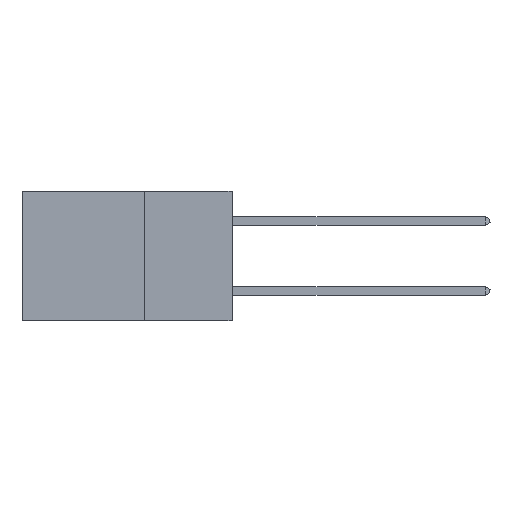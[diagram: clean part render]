
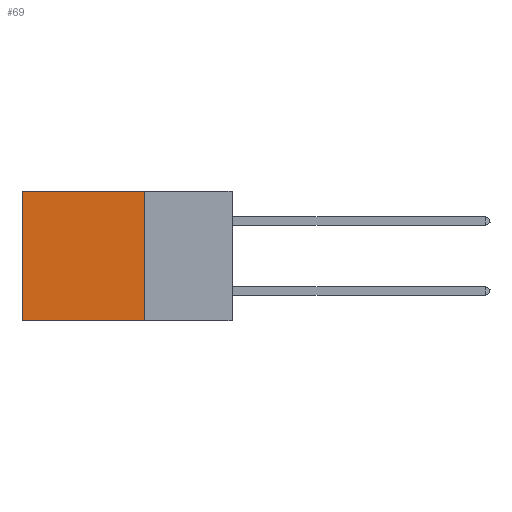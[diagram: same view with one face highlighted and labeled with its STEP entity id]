
A CAD part, left-side view. The second image highlights one B-rep face of the part: STEP entity #69.
In plain terms, the highlighted planar face has unit normal (-1, 0, 0).
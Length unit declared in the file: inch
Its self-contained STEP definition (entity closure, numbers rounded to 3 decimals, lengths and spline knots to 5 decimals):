
#69 = ADVANCED_FACE ( 'NONE', ( #638 ), #16818, .F. ) ;
#638 = FACE_OUTER_BOUND ( 'NONE', #28349, .T. ) ;
#1657 = VECTOR ( 'NONE', #23909, 39.37008 ) ;
#3343 = CARTESIAN_POINT ( 'NONE',  ( 0.2875, 0.25, -0.37 ) ) ;
#3465 = ORIENTED_EDGE ( 'NONE', *, *, #26536, .F. ) ;
#4228 = LINE ( 'NONE', #7484, #1657 ) ;
#5165 = EDGE_CURVE ( 'NONE', #7110, #7031, #12620, .T. ) ;
#7031 = VERTEX_POINT ( 'NONE', #13785 ) ;
#7110 = VERTEX_POINT ( 'NONE', #11536 ) ;
#7484 = CARTESIAN_POINT ( 'NONE',  ( 0.2875, 0.25, 0. ) ) ;
#7607 = ORIENTED_EDGE ( 'NONE', *, *, #5165, .T. ) ;
#9063 = ORIENTED_EDGE ( 'NONE', *, *, #27672, .F. ) ;
#9818 = AXIS2_PLACEMENT_3D ( 'NONE', #23804, #14626, #26576 ) ;
#10009 = DIRECTION ( 'NONE',  ( 0., 0., -1. ) ) ;
#11536 = CARTESIAN_POINT ( 'NONE',  ( 0.2875, 0.6, 0. ) ) ;
#11540 = VECTOR ( 'NONE', #24795, 39.37008 ) ;
#12210 = CARTESIAN_POINT ( 'NONE',  ( 0.2875, 0.25, 0. ) ) ;
#12338 = ORIENTED_EDGE ( 'NONE', *, *, #17400, .T. ) ;
#12620 = LINE ( 'NONE', #28784, #22590 ) ;
#13785 = CARTESIAN_POINT ( 'NONE',  ( 0.2875, 0.6, -0.37 ) ) ;
#14049 = CARTESIAN_POINT ( 'NONE',  ( 0.2875, 0.25, -0.37 ) ) ;
#14626 = DIRECTION ( 'NONE',  ( 1., 0., 0. ) ) ;
#14681 = CARTESIAN_POINT ( 'NONE',  ( 0.2875, 0.25, 0. ) ) ;
#16118 = DIRECTION ( 'NONE',  ( 0., 1., 0. ) ) ;
#16330 = LINE ( 'NONE', #14681, #20383 ) ;
#16818 = PLANE ( 'NONE',  #9818 ) ;
#17400 = EDGE_CURVE ( 'NONE', #18051, #7110, #16330, .T. ) ;
#18051 = VERTEX_POINT ( 'NONE', #12210 ) ;
#20383 = VECTOR ( 'NONE', #16118, 39.37008 ) ;
#22590 = VECTOR ( 'NONE', #10009, 39.37008 ) ;
#22954 = VERTEX_POINT ( 'NONE', #14049 ) ;
#23804 = CARTESIAN_POINT ( 'NONE',  ( 0.2875, 0.25, 0. ) ) ;
#23909 = DIRECTION ( 'NONE',  ( 0., 0., -1. ) ) ;
#24051 = LINE ( 'NONE', #3343, #11540 ) ;
#24795 = DIRECTION ( 'NONE',  ( 0., 1., 0. ) ) ;
#26536 = EDGE_CURVE ( 'NONE', #22954, #7031, #24051, .T. ) ;
#26576 = DIRECTION ( 'NONE',  ( 0., 0., -1. ) ) ;
#27672 = EDGE_CURVE ( 'NONE', #18051, #22954, #4228, .T. ) ;
#28349 = EDGE_LOOP ( 'NONE', ( #7607, #3465, #9063, #12338 ) ) ;
#28784 = CARTESIAN_POINT ( 'NONE',  ( 0.2875, 0.6, 0. ) ) ;
